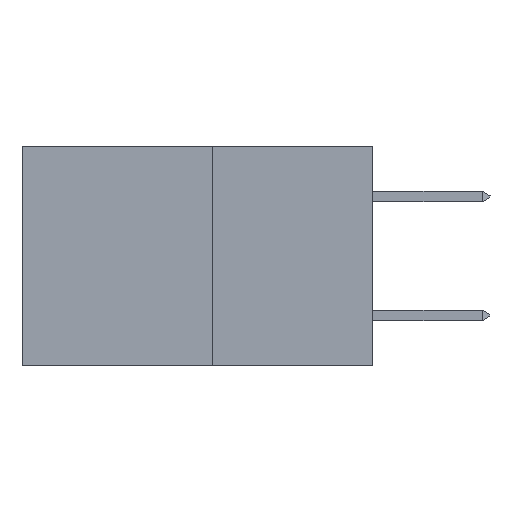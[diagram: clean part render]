
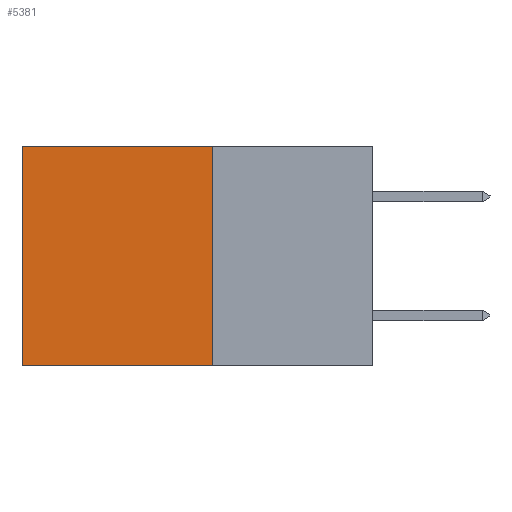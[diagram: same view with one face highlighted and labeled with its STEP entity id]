
A CAD part, left-side view. The second image highlights one B-rep face of the part: STEP entity #5381.
In plain terms, the highlighted planar face has unit normal (-1, 0, 0).
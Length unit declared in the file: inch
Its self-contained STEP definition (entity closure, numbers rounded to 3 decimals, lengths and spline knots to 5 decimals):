
#59 = CARTESIAN_POINT ( 'NONE',  ( 0.277, 0.59, -0.37 ) ) ;
#91 = DIRECTION ( 'NONE',  ( 0., 0., -1. ) ) ;
#579 = VERTEX_POINT ( 'NONE', #1889 ) ;
#837 = CARTESIAN_POINT ( 'NONE',  ( 0.277, 0.27, -0.37 ) ) ;
#893 = CARTESIAN_POINT ( 'NONE',  ( 0.277, 0.27, 0. ) ) ;
#1086 = ORIENTED_EDGE ( 'NONE', *, *, #7866, .F. ) ;
#1748 = VERTEX_POINT ( 'NONE', #3708 ) ;
#1889 = CARTESIAN_POINT ( 'NONE',  ( 0.277, 0.27, 0. ) ) ;
#2111 = CARTESIAN_POINT ( 'NONE',  ( 0.277, 0.27, -0.37 ) ) ;
#2118 = VECTOR ( 'NONE', #7495, 39.37008 ) ;
#2146 = CARTESIAN_POINT ( 'NONE',  ( 0.277, 0.27, -0.37 ) ) ;
#2913 = DIRECTION ( 'NONE',  ( 0., 0., -1. ) ) ;
#3262 = EDGE_CURVE ( 'NONE', #6757, #1748, #6462, .T. ) ;
#3375 = DIRECTION ( 'NONE',  ( 0., 1., 0. ) ) ;
#3436 = VERTEX_POINT ( 'NONE', #8717 ) ;
#3642 = PLANE ( 'NONE',  #5666 ) ;
#3659 = LINE ( 'NONE', #6770, #2118 ) ;
#3708 = CARTESIAN_POINT ( 'NONE',  ( 0.277, 0.59, -0.37 ) ) ;
#3969 = VECTOR ( 'NONE', #91, 39.37008 ) ;
#4224 = LINE ( 'NONE', #893, #7709 ) ;
#4441 = VECTOR ( 'NONE', #3375, 39.37008 ) ;
#4919 = EDGE_CURVE ( 'NONE', #3436, #1748, #5958, .T. ) ;
#5381 = ADVANCED_FACE ( 'NONE', ( #8134 ), #3642, .F. ) ;
#5666 = AXIS2_PLACEMENT_3D ( 'NONE', #2146, #7365, #2913 ) ;
#5958 = LINE ( 'NONE', #59, #3969 ) ;
#6187 = ORIENTED_EDGE ( 'NONE', *, *, #4919, .T. ) ;
#6462 = LINE ( 'NONE', #2111, #4441 ) ;
#6757 = VERTEX_POINT ( 'NONE', #837 ) ;
#6770 = CARTESIAN_POINT ( 'NONE',  ( 0.277, 0.27, -0.37 ) ) ;
#7358 = EDGE_LOOP ( 'NONE', ( #6187, #9184, #1086, #8750 ) ) ;
#7365 = DIRECTION ( 'NONE',  ( 1., 0., 0. ) ) ;
#7495 = DIRECTION ( 'NONE',  ( 0., 0., -1. ) ) ;
#7652 = DIRECTION ( 'NONE',  ( 0., 1., 0. ) ) ;
#7709 = VECTOR ( 'NONE', #7652, 39.37008 ) ;
#7866 = EDGE_CURVE ( 'NONE', #579, #6757, #3659, .T. ) ;
#8043 = EDGE_CURVE ( 'NONE', #579, #3436, #4224, .T. ) ;
#8134 = FACE_OUTER_BOUND ( 'NONE', #7358, .T. ) ;
#8717 = CARTESIAN_POINT ( 'NONE',  ( 0.277, 0.59, 0. ) ) ;
#8750 = ORIENTED_EDGE ( 'NONE', *, *, #8043, .T. ) ;
#9184 = ORIENTED_EDGE ( 'NONE', *, *, #3262, .F. ) ;
